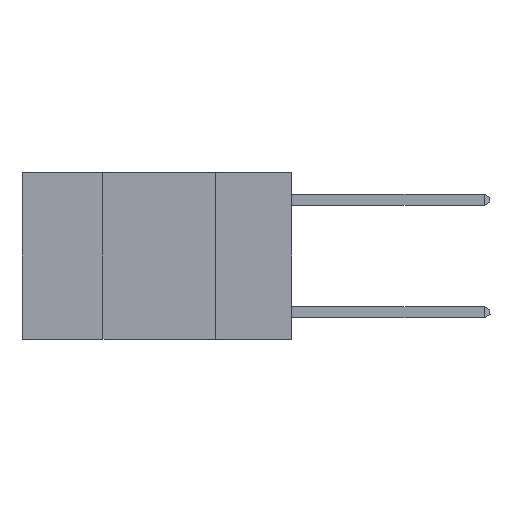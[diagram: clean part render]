
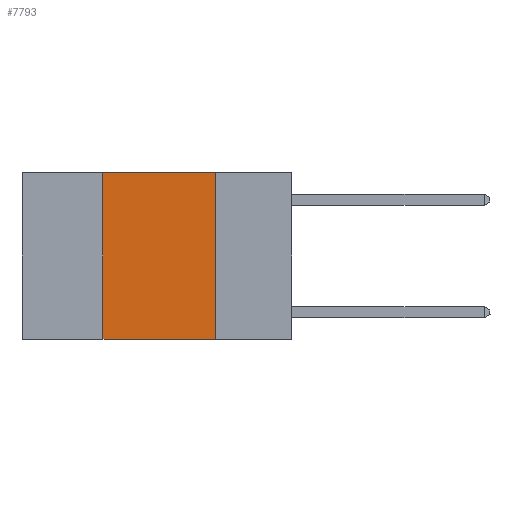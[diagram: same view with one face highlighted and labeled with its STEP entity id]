
A CAD part, left-side view. The second image highlights one B-rep face of the part: STEP entity #7793.
In plain terms, the highlighted planar face has unit normal (-1, 0, 0).
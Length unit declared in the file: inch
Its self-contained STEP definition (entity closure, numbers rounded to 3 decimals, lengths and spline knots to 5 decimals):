
#187 = LINE ( 'NONE', #7506, #6402 ) ;
#621 = CARTESIAN_POINT ( 'NONE',  ( 0., 0.6, 0. ) ) ;
#701 = CARTESIAN_POINT ( 'NONE',  ( 0., 0.17, 0. ) ) ;
#904 = ORIENTED_EDGE ( 'NONE', *, *, #7806, .F. ) ;
#2214 = EDGE_CURVE ( 'NONE', #6538, #4310, #10067, .T. ) ;
#3844 = LINE ( 'NONE', #9100, #7280 ) ;
#3951 = DIRECTION ( 'NONE',  ( 0., -1., 0. ) ) ;
#3999 = CARTESIAN_POINT ( 'NONE',  ( 0., 0.42, -0.37 ) ) ;
#4186 = CARTESIAN_POINT ( 'NONE',  ( 0., 0.17, 0. ) ) ;
#4310 = VERTEX_POINT ( 'NONE', #6134 ) ;
#4716 = VERTEX_POINT ( 'NONE', #9685 ) ;
#4788 = AXIS2_PLACEMENT_3D ( 'NONE', #621, #9867, #10659 ) ;
#4992 = ORIENTED_EDGE ( 'NONE', *, *, #9542, .F. ) ;
#5519 = FACE_OUTER_BOUND ( 'NONE', #9634, .T. ) ;
#6026 = DIRECTION ( 'NONE',  ( 0., 0., 1. ) ) ;
#6134 = CARTESIAN_POINT ( 'NONE',  ( 0., 0.17, -0.37 ) ) ;
#6281 = ORIENTED_EDGE ( 'NONE', *, *, #2214, .F. ) ;
#6402 = VECTOR ( 'NONE', #9321, 39.37008 ) ;
#6538 = VERTEX_POINT ( 'NONE', #4186 ) ;
#6606 = VECTOR ( 'NONE', #6026, 39.37008 ) ;
#6839 = LINE ( 'NONE', #10210, #6606 ) ;
#7069 = VECTOR ( 'NONE', #7527, 39.37008 ) ;
#7280 = VECTOR ( 'NONE', #3951, 39.37008 ) ;
#7467 = EDGE_CURVE ( 'NONE', #7771, #4310, #187, .T. ) ;
#7506 = CARTESIAN_POINT ( 'NONE',  ( 0., 0.6, -0.37 ) ) ;
#7527 = DIRECTION ( 'NONE',  ( 0., 0., -1. ) ) ;
#7682 = ORIENTED_EDGE ( 'NONE', *, *, #7467, .T. ) ;
#7771 = VERTEX_POINT ( 'NONE', #3999 ) ;
#7793 = ADVANCED_FACE ( 'NONE', ( #5519 ), #8131, .F. ) ;
#7806 = EDGE_CURVE ( 'NONE', #4716, #6538, #3844, .T. ) ;
#8131 = PLANE ( 'NONE',  #4788 ) ;
#9100 = CARTESIAN_POINT ( 'NONE',  ( 0., 0.6, 0. ) ) ;
#9321 = DIRECTION ( 'NONE',  ( 0., -1., 0. ) ) ;
#9542 = EDGE_CURVE ( 'NONE', #7771, #4716, #6839, .T. ) ;
#9634 = EDGE_LOOP ( 'NONE', ( #6281, #904, #4992, #7682 ) ) ;
#9685 = CARTESIAN_POINT ( 'NONE',  ( 0., 0.42, 0. ) ) ;
#9867 = DIRECTION ( 'NONE',  ( 1., 0., 0. ) ) ;
#10067 = LINE ( 'NONE', #701, #7069 ) ;
#10210 = CARTESIAN_POINT ( 'NONE',  ( 0., 0.42, 0. ) ) ;
#10659 = DIRECTION ( 'NONE',  ( 0., 0., -1. ) ) ;
